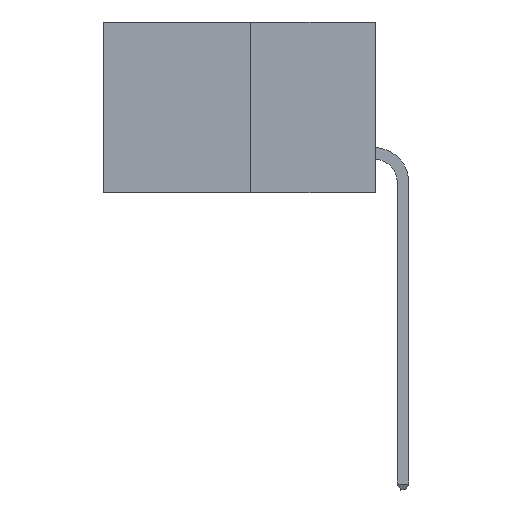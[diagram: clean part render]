
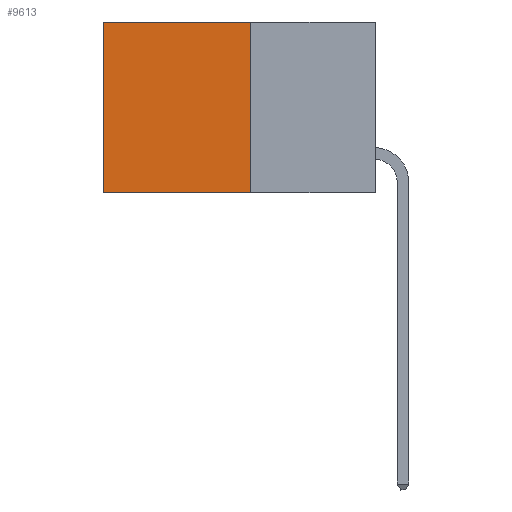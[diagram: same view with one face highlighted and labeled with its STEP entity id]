
A CAD part, left-side view. The second image highlights one B-rep face of the part: STEP entity #9613.
In plain terms, the highlighted planar face has unit normal (-1, 0, 0).
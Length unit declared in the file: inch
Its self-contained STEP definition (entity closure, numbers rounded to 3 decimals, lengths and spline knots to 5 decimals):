
#565 = EDGE_LOOP ( 'NONE', ( #718, #25352, #1196, #24123 ) ) ;
#718 = ORIENTED_EDGE ( 'NONE', *, *, #23443, .T. ) ;
#791 = CARTESIAN_POINT ( 'NONE',  ( 0.277, 0.59, 0. ) ) ;
#1196 = ORIENTED_EDGE ( 'NONE', *, *, #15557, .F. ) ;
#2774 = VECTOR ( 'NONE', #16930, 39.37008 ) ;
#2812 = DIRECTION ( 'NONE',  ( 0., 1., 0. ) ) ;
#3268 = FACE_OUTER_BOUND ( 'NONE', #565, .T. ) ;
#3515 = CARTESIAN_POINT ( 'NONE',  ( 0.277, 0.59, -0.37 ) ) ;
#5182 = LINE ( 'NONE', #20379, #30249 ) ;
#7586 = PLANE ( 'NONE',  #12780 ) ;
#7895 = DIRECTION ( 'NONE',  ( 0., 0., -1. ) ) ;
#9613 = ADVANCED_FACE ( 'NONE', ( #3268 ), #7586, .F. ) ;
#10119 = CARTESIAN_POINT ( 'NONE',  ( 0.277, 0.27, 0. ) ) ;
#10129 = DIRECTION ( 'NONE',  ( 0., 0., -1. ) ) ;
#12780 = AXIS2_PLACEMENT_3D ( 'NONE', #15018, #25108, #10129 ) ;
#13141 = VECTOR ( 'NONE', #2812, 39.37008 ) ;
#14305 = VERTEX_POINT ( 'NONE', #27706 ) ;
#15018 = CARTESIAN_POINT ( 'NONE',  ( 0.277, 0.27, -0.37 ) ) ;
#15557 = EDGE_CURVE ( 'NONE', #16709, #23515, #5182, .T. ) ;
#16709 = VERTEX_POINT ( 'NONE', #10119 ) ;
#16930 = DIRECTION ( 'NONE',  ( 0., 1., 0. ) ) ;
#18824 = VERTEX_POINT ( 'NONE', #791 ) ;
#20379 = CARTESIAN_POINT ( 'NONE',  ( 0.277, 0.27, -0.37 ) ) ;
#20392 = CARTESIAN_POINT ( 'NONE',  ( 0.277, 0.27, 0. ) ) ;
#21092 = DIRECTION ( 'NONE',  ( 0., 0., -1. ) ) ;
#21960 = CARTESIAN_POINT ( 'NONE',  ( 0.277, 0.27, -0.37 ) ) ;
#22815 = LINE ( 'NONE', #21960, #2774 ) ;
#23443 = EDGE_CURVE ( 'NONE', #18824, #14305, #26154, .T. ) ;
#23515 = VERTEX_POINT ( 'NONE', #28698 ) ;
#24123 = ORIENTED_EDGE ( 'NONE', *, *, #24460, .T. ) ;
#24460 = EDGE_CURVE ( 'NONE', #16709, #18824, #26463, .T. ) ;
#25108 = DIRECTION ( 'NONE',  ( 1., 0., 0. ) ) ;
#25352 = ORIENTED_EDGE ( 'NONE', *, *, #31010, .F. ) ;
#26154 = LINE ( 'NONE', #3515, #26918 ) ;
#26463 = LINE ( 'NONE', #20392, #13141 ) ;
#26918 = VECTOR ( 'NONE', #21092, 39.37008 ) ;
#27706 = CARTESIAN_POINT ( 'NONE',  ( 0.277, 0.59, -0.37 ) ) ;
#28698 = CARTESIAN_POINT ( 'NONE',  ( 0.277, 0.27, -0.37 ) ) ;
#30249 = VECTOR ( 'NONE', #7895, 39.37008 ) ;
#31010 = EDGE_CURVE ( 'NONE', #23515, #14305, #22815, .T. ) ;
